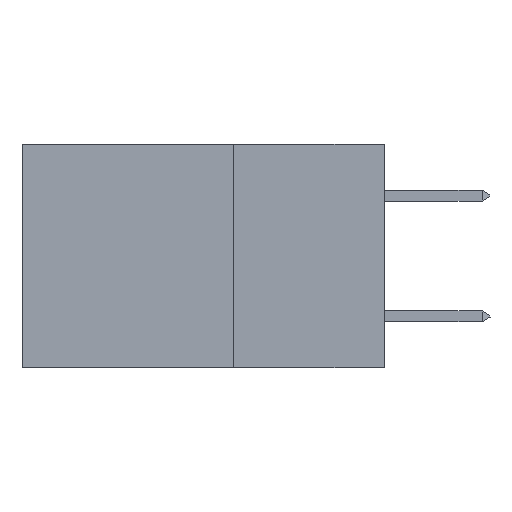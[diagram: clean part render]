
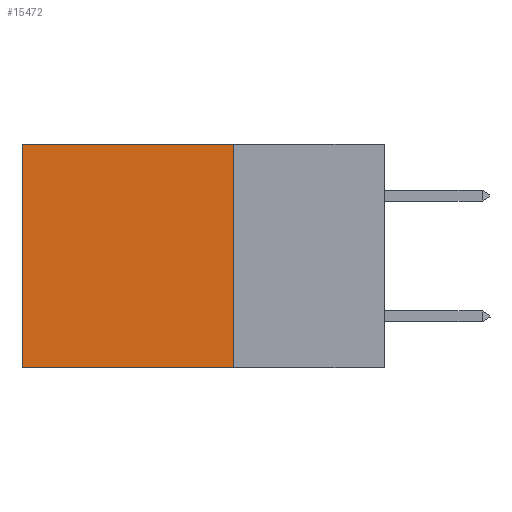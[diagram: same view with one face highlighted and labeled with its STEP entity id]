
A CAD part, left-side view. The second image highlights one B-rep face of the part: STEP entity #15472.
In plain terms, the highlighted planar face has unit normal (-1, 0, 0).
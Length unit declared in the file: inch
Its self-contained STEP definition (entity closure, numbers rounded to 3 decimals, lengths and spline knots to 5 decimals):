
#22 = DIRECTION ( 'NONE',  ( 0., 1., 0. ) ) ;
#272 = CARTESIAN_POINT ( 'NONE',  ( 0.2875, 0.25, -0.37 ) ) ;
#627 = CARTESIAN_POINT ( 'NONE',  ( 0.2875, 0.6, 0. ) ) ;
#934 = DIRECTION ( 'NONE',  ( 1., 0., 0. ) ) ;
#2937 = DIRECTION ( 'NONE',  ( 0., 0., -1. ) ) ;
#3008 = CARTESIAN_POINT ( 'NONE',  ( 0.2875, 0.6, 0. ) ) ;
#3056 = VERTEX_POINT ( 'NONE', #8049 ) ;
#3119 = VECTOR ( 'NONE', #14769, 39.37008 ) ;
#3721 = ORIENTED_EDGE ( 'NONE', *, *, #4991, .F. ) ;
#4369 = LINE ( 'NONE', #627, #3119 ) ;
#4991 = EDGE_CURVE ( 'NONE', #18350, #3056, #14512, .T. ) ;
#5268 = EDGE_CURVE ( 'NONE', #16018, #7866, #4369, .T. ) ;
#7478 = ORIENTED_EDGE ( 'NONE', *, *, #5268, .T. ) ;
#7866 = VERTEX_POINT ( 'NONE', #8167 ) ;
#8049 = CARTESIAN_POINT ( 'NONE',  ( 0.2875, 0.25, -0.37 ) ) ;
#8167 = CARTESIAN_POINT ( 'NONE',  ( 0.2875, 0.6, -0.37 ) ) ;
#8476 = LINE ( 'NONE', #19744, #16005 ) ;
#9083 = CARTESIAN_POINT ( 'NONE',  ( 0.2875, 0.25, 0. ) ) ;
#10204 = EDGE_CURVE ( 'NONE', #18350, #16018, #8476, .T. ) ;
#10268 = EDGE_CURVE ( 'NONE', #3056, #7866, #13803, .T. ) ;
#10709 = PLANE ( 'NONE',  #13305 ) ;
#10974 = CARTESIAN_POINT ( 'NONE',  ( 0.2875, 0.25, 0. ) ) ;
#11687 = VECTOR ( 'NONE', #21807, 39.37008 ) ;
#11725 = CARTESIAN_POINT ( 'NONE',  ( 0.2875, 0.25, 0. ) ) ;
#12452 = EDGE_LOOP ( 'NONE', ( #7478, #24061, #3721, #25467 ) ) ;
#13190 = VECTOR ( 'NONE', #22, 39.37008 ) ;
#13305 = AXIS2_PLACEMENT_3D ( 'NONE', #10974, #934, #2937 ) ;
#13803 = LINE ( 'NONE', #272, #13190 ) ;
#14512 = LINE ( 'NONE', #11725, #11687 ) ;
#14636 = FACE_OUTER_BOUND ( 'NONE', #12452, .T. ) ;
#14769 = DIRECTION ( 'NONE',  ( 0., 0., -1. ) ) ;
#15472 = ADVANCED_FACE ( 'NONE', ( #14636 ), #10709, .F. ) ;
#16005 = VECTOR ( 'NONE', #23758, 39.37008 ) ;
#16018 = VERTEX_POINT ( 'NONE', #3008 ) ;
#18350 = VERTEX_POINT ( 'NONE', #9083 ) ;
#19744 = CARTESIAN_POINT ( 'NONE',  ( 0.2875, 0.25, 0. ) ) ;
#21807 = DIRECTION ( 'NONE',  ( 0., 0., -1. ) ) ;
#23758 = DIRECTION ( 'NONE',  ( 0., 1., 0. ) ) ;
#24061 = ORIENTED_EDGE ( 'NONE', *, *, #10268, .F. ) ;
#25467 = ORIENTED_EDGE ( 'NONE', *, *, #10204, .T. ) ;
